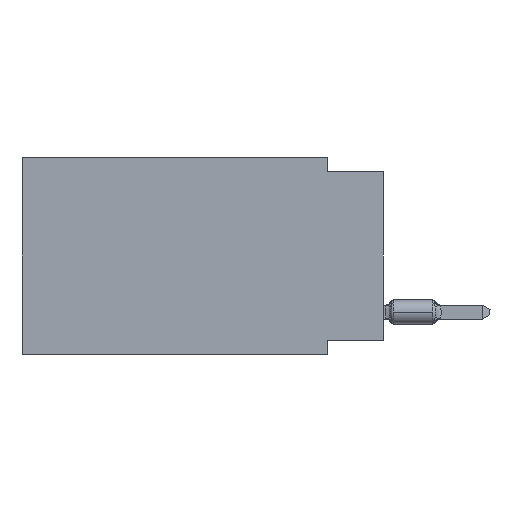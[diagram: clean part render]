
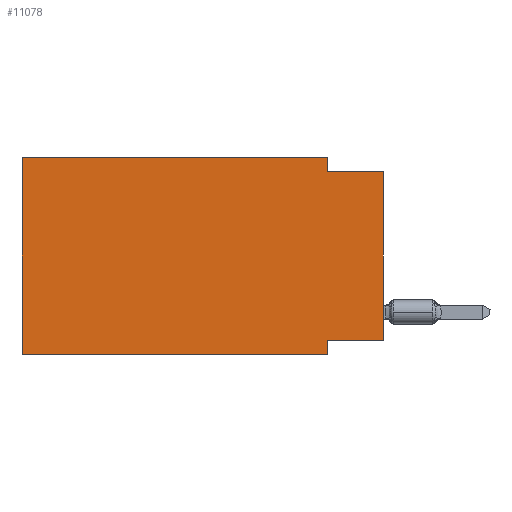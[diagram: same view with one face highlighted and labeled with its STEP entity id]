
A CAD part, left-side view. The second image highlights one B-rep face of the part: STEP entity #11078.
In plain terms, the highlighted planar face has unit normal (-1, 0, 0).
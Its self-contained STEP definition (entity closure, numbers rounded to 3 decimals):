
#358 = VERTEX_POINT ( 'NONE', #13789 ) ;
#722 = EDGE_CURVE ( 'NONE', #9185, #24776, #25551, .T. ) ;
#825 = DIRECTION ( 'NONE',  ( 0., -1., 0. ) ) ;
#1595 = VECTOR ( 'NONE', #14334, 1000. ) ;
#2269 = ORIENTED_EDGE ( 'NONE', *, *, #11488, .F. ) ;
#2394 = CARTESIAN_POINT ( 'NONE',  ( 0., 16.383, 0. ) ) ;
#2801 = CARTESIAN_POINT ( 'NONE',  ( 0., 16.383, 0. ) ) ;
#2900 = ORIENTED_EDGE ( 'NONE', *, *, #28456, .F. ) ;
#3448 = CARTESIAN_POINT ( 'NONE',  ( 0., 0., -0.635 ) ) ;
#3711 = CARTESIAN_POINT ( 'NONE',  ( 0., 0., -0.635 ) ) ;
#4990 = PLANE ( 'NONE',  #28212 ) ;
#6199 = CARTESIAN_POINT ( 'NONE',  ( 0., 16.383, -8.89 ) ) ;
#6669 = LINE ( 'NONE', #19846, #23778 ) ;
#8387 = LINE ( 'NONE', #6199, #18680 ) ;
#8515 = CARTESIAN_POINT ( 'NONE',  ( 0., 2.54, 0. ) ) ;
#8604 = ORIENTED_EDGE ( 'NONE', *, *, #12043, .F. ) ;
#8809 = VECTOR ( 'NONE', #27461, 1000. ) ;
#9185 = VERTEX_POINT ( 'NONE', #8515 ) ;
#10377 = LINE ( 'NONE', #16388, #27222 ) ;
#11078 = ADVANCED_FACE ( 'NONE', ( #25180 ), #4990, .F. ) ;
#11210 = VERTEX_POINT ( 'NONE', #3711 ) ;
#11254 = ORIENTED_EDGE ( 'NONE', *, *, #17573, .T. ) ;
#11488 = EDGE_CURVE ( 'NONE', #21120, #9185, #15704, .T. ) ;
#11669 = CARTESIAN_POINT ( 'NONE',  ( 0., 0., 0. ) ) ;
#11731 = DIRECTION ( 'NONE',  ( 1., 0., 0. ) ) ;
#11756 = VERTEX_POINT ( 'NONE', #18260 ) ;
#11872 = CARTESIAN_POINT ( 'NONE',  ( 0., 0., -8.255 ) ) ;
#12043 = EDGE_CURVE ( 'NONE', #12756, #17275, #6669, .T. ) ;
#12331 = ORIENTED_EDGE ( 'NONE', *, *, #722, .F. ) ;
#12756 = VERTEX_POINT ( 'NONE', #27847 ) ;
#13141 = VECTOR ( 'NONE', #27471, 1000. ) ;
#13364 = DIRECTION ( 'NONE',  ( 0., -1., 0. ) ) ;
#13399 = DIRECTION ( 'NONE',  ( 0., 0., -1. ) ) ;
#13789 = CARTESIAN_POINT ( 'NONE',  ( 0., 0., -8.255 ) ) ;
#14334 = DIRECTION ( 'NONE',  ( 0., 1., 0. ) ) ;
#15704 = LINE ( 'NONE', #2394, #28929 ) ;
#15958 = EDGE_CURVE ( 'NONE', #11756, #17275, #8387, .T. ) ;
#16208 = LINE ( 'NONE', #11669, #13141 ) ;
#16388 = CARTESIAN_POINT ( 'NONE',  ( 0., 16.383, 0. ) ) ;
#16682 = LINE ( 'NONE', #11872, #1595 ) ;
#17043 = DIRECTION ( 'NONE',  ( 0., -1., 0. ) ) ;
#17275 = VERTEX_POINT ( 'NONE', #18868 ) ;
#17573 = EDGE_CURVE ( 'NONE', #358, #11210, #16208, .T. ) ;
#17758 = ORIENTED_EDGE ( 'NONE', *, *, #15958, .T. ) ;
#18219 = VECTOR ( 'NONE', #825, 1000. ) ;
#18260 = CARTESIAN_POINT ( 'NONE',  ( 0., 16.383, -8.89 ) ) ;
#18680 = VECTOR ( 'NONE', #17043, 1000. ) ;
#18863 = EDGE_LOOP ( 'NONE', ( #11254, #23364, #12331, #2269, #2900, #17758, #8604, #22364 ) ) ;
#18868 = CARTESIAN_POINT ( 'NONE',  ( 0., 2.54, -8.89 ) ) ;
#18960 = EDGE_CURVE ( 'NONE', #24776, #11210, #27458, .T. ) ;
#19846 = CARTESIAN_POINT ( 'NONE',  ( 0., 2.54, -8.89 ) ) ;
#20652 = DIRECTION ( 'NONE',  ( 0., 0., -1. ) ) ;
#21120 = VERTEX_POINT ( 'NONE', #28706 ) ;
#22364 = ORIENTED_EDGE ( 'NONE', *, *, #23706, .F. ) ;
#23329 = CARTESIAN_POINT ( 'NONE',  ( 0., 2.54, 0. ) ) ;
#23364 = ORIENTED_EDGE ( 'NONE', *, *, #18960, .F. ) ;
#23706 = EDGE_CURVE ( 'NONE', #358, #12756, #16682, .T. ) ;
#23778 = VECTOR ( 'NONE', #13399, 1000. ) ;
#24776 = VERTEX_POINT ( 'NONE', #28014 ) ;
#25180 = FACE_OUTER_BOUND ( 'NONE', #18863, .T. ) ;
#25551 = LINE ( 'NONE', #23329, #8809 ) ;
#27222 = VECTOR ( 'NONE', #27814, 1000. ) ;
#27458 = LINE ( 'NONE', #3448, #18219 ) ;
#27461 = DIRECTION ( 'NONE',  ( 0., 0., -1. ) ) ;
#27471 = DIRECTION ( 'NONE',  ( 0., 0., 1. ) ) ;
#27814 = DIRECTION ( 'NONE',  ( 0., 0., 1. ) ) ;
#27847 = CARTESIAN_POINT ( 'NONE',  ( 0., 2.54, -8.255 ) ) ;
#28014 = CARTESIAN_POINT ( 'NONE',  ( 0., 2.54, -0.635 ) ) ;
#28212 = AXIS2_PLACEMENT_3D ( 'NONE', #2801, #11731, #20652 ) ;
#28456 = EDGE_CURVE ( 'NONE', #11756, #21120, #10377, .T. ) ;
#28706 = CARTESIAN_POINT ( 'NONE',  ( 0., 16.383, 0. ) ) ;
#28929 = VECTOR ( 'NONE', #13364, 1000. ) ;
